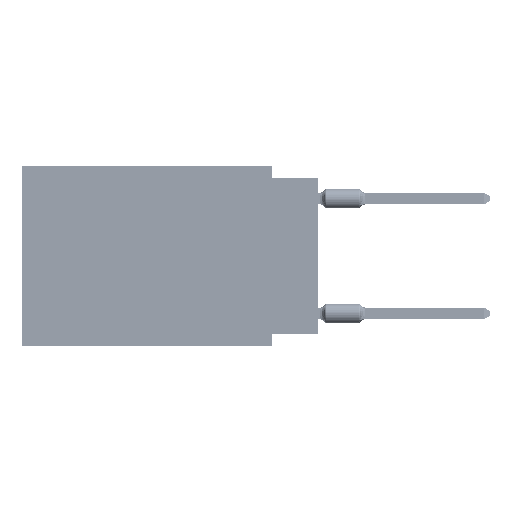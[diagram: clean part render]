
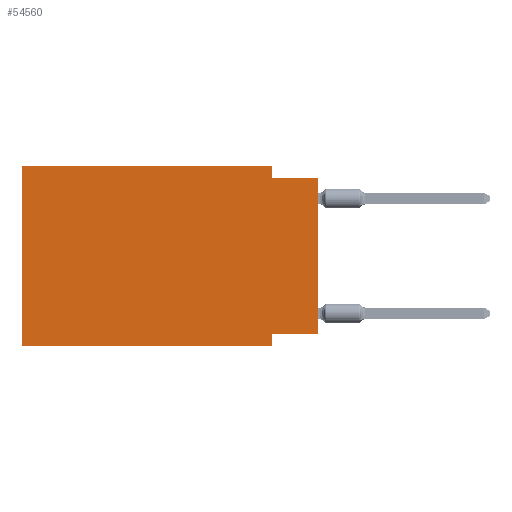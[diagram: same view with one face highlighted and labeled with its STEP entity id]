
A CAD part, left-side view. The second image highlights one B-rep face of the part: STEP entity #54560.
In plain terms, the highlighted planar face has unit normal (-1, 0, 0).
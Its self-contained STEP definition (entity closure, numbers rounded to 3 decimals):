
#36 = LINE ( 'NONE', #11224, #50827 ) ;
#1039 = EDGE_CURVE ( 'NONE', #2034, #26926, #29941, .T. ) ;
#1209 = CARTESIAN_POINT ( 'NONE',  ( 0., 0., 0. ) ) ;
#2034 = VERTEX_POINT ( 'NONE', #62060 ) ;
#5235 = EDGE_CURVE ( 'NONE', #58037, #76782, #64287, .T. ) ;
#6074 = ORIENTED_EDGE ( 'NONE', *, *, #52367, .F. ) ;
#6268 = CARTESIAN_POINT ( 'NONE',  ( 0., 16.383, 0. ) ) ;
#7965 = LINE ( 'NONE', #1209, #10097 ) ;
#9596 = FACE_OUTER_BOUND ( 'NONE', #12513, .T. ) ;
#10097 = VECTOR ( 'NONE', #62995, 1000. ) ;
#10885 = VERTEX_POINT ( 'NONE', #64304 ) ;
#11224 = CARTESIAN_POINT ( 'NONE',  ( 0., 0., -9.271 ) ) ;
#12513 = EDGE_LOOP ( 'NONE', ( #71436, #38918, #19452, #6074, #24861, #49380, #61040, #23519 ) ) ;
#13839 = EDGE_CURVE ( 'NONE', #26926, #50525, #37595, .T. ) ;
#15221 = LINE ( 'NONE', #75855, #57386 ) ;
#16886 = DIRECTION ( 'NONE',  ( 0., -1., 0. ) ) ;
#17468 = LINE ( 'NONE', #6268, #29803 ) ;
#18211 = VECTOR ( 'NONE', #48291, 1000. ) ;
#19452 = ORIENTED_EDGE ( 'NONE', *, *, #1039, .F. ) ;
#21597 = CARTESIAN_POINT ( 'NONE',  ( 0., 2.54, -9.906 ) ) ;
#22343 = CARTESIAN_POINT ( 'NONE',  ( 0., 16.383, 0. ) ) ;
#23027 = DIRECTION ( 'NONE',  ( 0., 0., 1. ) ) ;
#23342 = CARTESIAN_POINT ( 'NONE',  ( 0., 0., -9.271 ) ) ;
#23519 = ORIENTED_EDGE ( 'NONE', *, *, #72251, .F. ) ;
#24340 = DIRECTION ( 'NONE',  ( 0., 1., 0. ) ) ;
#24861 = ORIENTED_EDGE ( 'NONE', *, *, #31689, .F. ) ;
#26926 = VERTEX_POINT ( 'NONE', #78360 ) ;
#27921 = PLANE ( 'NONE',  #41913 ) ;
#29803 = VECTOR ( 'NONE', #23027, 1000. ) ;
#29941 = LINE ( 'NONE', #43498, #18211 ) ;
#31689 = EDGE_CURVE ( 'NONE', #57632, #10885, #17468, .T. ) ;
#36976 = CARTESIAN_POINT ( 'NONE',  ( 0., 0., -0.635 ) ) ;
#37595 = LINE ( 'NONE', #51109, #66603 ) ;
#38918 = ORIENTED_EDGE ( 'NONE', *, *, #13839, .F. ) ;
#41913 = AXIS2_PLACEMENT_3D ( 'NONE', #22343, #52255, #76603 ) ;
#43498 = CARTESIAN_POINT ( 'NONE',  ( 0., 2.54, 0. ) ) ;
#44723 = VERTEX_POINT ( 'NONE', #23342 ) ;
#48291 = DIRECTION ( 'NONE',  ( 0., 0., -1. ) ) ;
#49380 = ORIENTED_EDGE ( 'NONE', *, *, #58271, .T. ) ;
#50525 = VERTEX_POINT ( 'NONE', #36976 ) ;
#50827 = VECTOR ( 'NONE', #24340, 1000. ) ;
#51109 = CARTESIAN_POINT ( 'NONE',  ( 0., 0., -0.635 ) ) ;
#52255 = DIRECTION ( 'NONE',  ( 1., 0., 0. ) ) ;
#52367 = EDGE_CURVE ( 'NONE', #10885, #2034, #78682, .T. ) ;
#54244 = VECTOR ( 'NONE', #16886, 1000. ) ;
#54560 = ADVANCED_FACE ( 'NONE', ( #9596 ), #27921, .F. ) ;
#57108 = DIRECTION ( 'NONE',  ( 0., -1., 0. ) ) ;
#57386 = VECTOR ( 'NONE', #57108, 1000. ) ;
#57632 = VERTEX_POINT ( 'NONE', #76540 ) ;
#58037 = VERTEX_POINT ( 'NONE', #59573 ) ;
#58271 = EDGE_CURVE ( 'NONE', #57632, #76782, #15221, .T. ) ;
#59573 = CARTESIAN_POINT ( 'NONE',  ( 0., 2.54, -9.271 ) ) ;
#61040 = ORIENTED_EDGE ( 'NONE', *, *, #5235, .F. ) ;
#62060 = CARTESIAN_POINT ( 'NONE',  ( 0., 2.54, 0. ) ) ;
#62995 = DIRECTION ( 'NONE',  ( 0., 0., 1. ) ) ;
#64287 = LINE ( 'NONE', #21597, #78505 ) ;
#64304 = CARTESIAN_POINT ( 'NONE',  ( 0., 16.383, 0. ) ) ;
#65076 = DIRECTION ( 'NONE',  ( 0., 0., -1. ) ) ;
#66603 = VECTOR ( 'NONE', #67936, 1000. ) ;
#67936 = DIRECTION ( 'NONE',  ( 0., -1., 0. ) ) ;
#71145 = CARTESIAN_POINT ( 'NONE',  ( 0., 16.383, 0. ) ) ;
#71436 = ORIENTED_EDGE ( 'NONE', *, *, #72347, .T. ) ;
#72251 = EDGE_CURVE ( 'NONE', #44723, #58037, #36, .T. ) ;
#72347 = EDGE_CURVE ( 'NONE', #44723, #50525, #7965, .T. ) ;
#75550 = CARTESIAN_POINT ( 'NONE',  ( 0., 2.54, -9.906 ) ) ;
#75855 = CARTESIAN_POINT ( 'NONE',  ( 0., 16.383, -9.906 ) ) ;
#76540 = CARTESIAN_POINT ( 'NONE',  ( 0., 16.383, -9.906 ) ) ;
#76603 = DIRECTION ( 'NONE',  ( 0., 0., -1. ) ) ;
#76782 = VERTEX_POINT ( 'NONE', #75550 ) ;
#78360 = CARTESIAN_POINT ( 'NONE',  ( 0., 2.54, -0.635 ) ) ;
#78505 = VECTOR ( 'NONE', #65076, 1000. ) ;
#78682 = LINE ( 'NONE', #71145, #54244 ) ;
